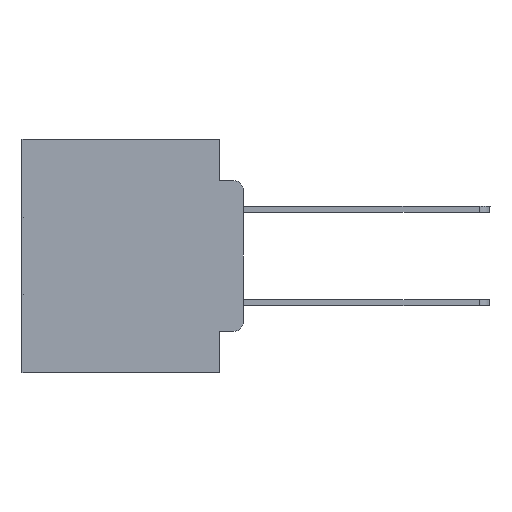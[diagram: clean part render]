
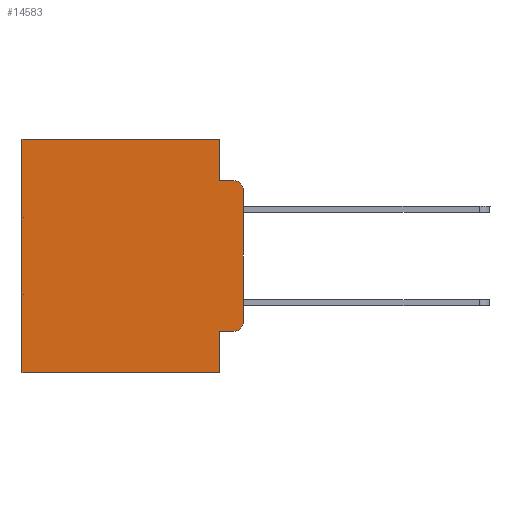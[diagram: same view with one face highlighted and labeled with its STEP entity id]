
A CAD part, left-side view. The second image highlights one B-rep face of the part: STEP entity #14583.
In plain terms, the highlighted planar face has unit normal (-1, 0, 0).
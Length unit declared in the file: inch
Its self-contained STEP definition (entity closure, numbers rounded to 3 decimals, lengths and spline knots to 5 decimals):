
#437 = ORIENTED_EDGE ( 'NONE', *, *, #23579, .T. ) ;
#608 = VECTOR ( 'NONE', #16041, 39.37008 ) ;
#628 = VERTEX_POINT ( 'NONE', #19815 ) ;
#632 = ORIENTED_EDGE ( 'NONE', *, *, #22511, .F. ) ;
#904 = LINE ( 'NONE', #3353, #23796 ) ;
#1685 = ORIENTED_EDGE ( 'NONE', *, *, #5824, .T. ) ;
#2234 = EDGE_CURVE ( 'NONE', #29441, #21208, #904, .T. ) ;
#2269 = ORIENTED_EDGE ( 'NONE', *, *, #23444, .F. ) ;
#2992 = LINE ( 'NONE', #22718, #5276 ) ;
#3216 = VERTEX_POINT ( 'NONE', #29055 ) ;
#3228 = VERTEX_POINT ( 'NONE', #14453 ) ;
#3332 = VERTEX_POINT ( 'NONE', #6909 ) ;
#3353 = CARTESIAN_POINT ( 'NONE',  ( 0.298, 0.051, 0. ) ) ;
#3535 = VECTOR ( 'NONE', #10659, 39.37008 ) ;
#3926 = DIRECTION ( 'NONE',  ( 1., 0., 0. ) ) ;
#4010 = CARTESIAN_POINT ( 'NONE',  ( 0.298, 0., -0.5 ) ) ;
#4019 = CIRCLE ( 'NONE', #18741, 0.02 ) ;
#4032 = CARTESIAN_POINT ( 'NONE',  ( 0.298, 0.02, -0.3915 ) ) ;
#4871 = VERTEX_POINT ( 'NONE', #31496 ) ;
#5253 = EDGE_CURVE ( 'NONE', #29441, #3228, #23105, .T. ) ;
#5276 = VECTOR ( 'NONE', #20769, 39.37008 ) ;
#5824 = EDGE_CURVE ( 'NONE', #3332, #26731, #4019, .T. ) ;
#6003 = DIRECTION ( 'NONE',  ( 0., 0., -1. ) ) ;
#6052 = DIRECTION ( 'NONE',  ( 0., 0., -1. ) ) ;
#6071 = EDGE_CURVE ( 'NONE', #3332, #23024, #2992, .T. ) ;
#6909 = CARTESIAN_POINT ( 'NONE',  ( 0.298, 0., -0.1085 ) ) ;
#7150 = EDGE_CURVE ( 'NONE', #628, #3216, #16087, .T. ) ;
#9857 = CIRCLE ( 'NONE', #19822, 0.02 ) ;
#10036 = ORIENTED_EDGE ( 'NONE', *, *, #7150, .T. ) ;
#10039 = CARTESIAN_POINT ( 'NONE',  ( 0.298, 0.051, -0.5 ) ) ;
#10659 = DIRECTION ( 'NONE',  ( 0., -1., 0. ) ) ;
#11721 = ORIENTED_EDGE ( 'NONE', *, *, #15536, .F. ) ;
#11780 = DIRECTION ( 'NONE',  ( -1., 0., 0. ) ) ;
#12861 = VECTOR ( 'NONE', #19102, 39.37008 ) ;
#13384 = LINE ( 'NONE', #28476, #12861 ) ;
#13494 = VECTOR ( 'NONE', #31547, 39.37008 ) ;
#13768 = DIRECTION ( 'NONE',  ( 0., 0., -1. ) ) ;
#13944 = ORIENTED_EDGE ( 'NONE', *, *, #2234, .F. ) ;
#14076 = VECTOR ( 'NONE', #16365, 39.37008 ) ;
#14153 = EDGE_LOOP ( 'NONE', ( #29452, #1685, #2269, #632, #18569, #10036, #11721, #13944, #29373, #437 ) ) ;
#14453 = CARTESIAN_POINT ( 'NONE',  ( 0.298, 0.02, -0.4115 ) ) ;
#14583 = ADVANCED_FACE ( 'NONE', ( #29064 ), #18916, .F. ) ;
#15536 = EDGE_CURVE ( 'NONE', #21208, #3216, #21444, .T. ) ;
#16041 = DIRECTION ( 'NONE',  ( 0., -1., 0. ) ) ;
#16087 = LINE ( 'NONE', #23145, #21070 ) ;
#16365 = DIRECTION ( 'NONE',  ( 0., 1., 0. ) ) ;
#18569 = ORIENTED_EDGE ( 'NONE', *, *, #20516, .T. ) ;
#18684 = CARTESIAN_POINT ( 'NONE',  ( 0.298, 0.051, -0.0885 ) ) ;
#18741 = AXIS2_PLACEMENT_3D ( 'NONE', #25905, #31010, #6052 ) ;
#18916 = PLANE ( 'NONE',  #28187 ) ;
#19102 = DIRECTION ( 'NONE',  ( 0., 1., 0. ) ) ;
#19372 = CARTESIAN_POINT ( 'NONE',  ( 0.298, 0., -0.3915 ) ) ;
#19815 = CARTESIAN_POINT ( 'NONE',  ( 0.298, 0.473, 0. ) ) ;
#19822 = AXIS2_PLACEMENT_3D ( 'NONE', #4032, #11780, #13768 ) ;
#20516 = EDGE_CURVE ( 'NONE', #4871, #628, #13384, .T. ) ;
#20769 = DIRECTION ( 'NONE',  ( 0., 0., -1. ) ) ;
#21070 = VECTOR ( 'NONE', #21168, 39.37008 ) ;
#21168 = DIRECTION ( 'NONE',  ( 0., 0., -1. ) ) ;
#21208 = VERTEX_POINT ( 'NONE', #10039 ) ;
#21444 = LINE ( 'NONE', #4010, #14076 ) ;
#22511 = EDGE_CURVE ( 'NONE', #4871, #27184, #29567, .T. ) ;
#22718 = CARTESIAN_POINT ( 'NONE',  ( 0.298, 0., 0. ) ) ;
#23024 = VERTEX_POINT ( 'NONE', #19372 ) ;
#23105 = LINE ( 'NONE', #26035, #608 ) ;
#23128 = LINE ( 'NONE', #23279, #3535 ) ;
#23145 = CARTESIAN_POINT ( 'NONE',  ( 0.298, 0.473, 0. ) ) ;
#23279 = CARTESIAN_POINT ( 'NONE',  ( 0.298, 0.051, -0.0885 ) ) ;
#23444 = EDGE_CURVE ( 'NONE', #27184, #26731, #23128, .T. ) ;
#23579 = EDGE_CURVE ( 'NONE', #3228, #23024, #9857, .T. ) ;
#23796 = VECTOR ( 'NONE', #6003, 39.37008 ) ;
#23811 = CARTESIAN_POINT ( 'NONE',  ( 0.298, 0., 0. ) ) ;
#25316 = CARTESIAN_POINT ( 'NONE',  ( 0.298, 0.051, -0.4115 ) ) ;
#25905 = CARTESIAN_POINT ( 'NONE',  ( 0.298, 0.02, -0.1085 ) ) ;
#26035 = CARTESIAN_POINT ( 'NONE',  ( 0.298, 0.051, -0.4115 ) ) ;
#26572 = CARTESIAN_POINT ( 'NONE',  ( 0.298, 0.02, -0.0885 ) ) ;
#26610 = CARTESIAN_POINT ( 'NONE',  ( 0.298, 0.051, 0. ) ) ;
#26731 = VERTEX_POINT ( 'NONE', #26572 ) ;
#27184 = VERTEX_POINT ( 'NONE', #18684 ) ;
#28187 = AXIS2_PLACEMENT_3D ( 'NONE', #23811, #3926, #28912 ) ;
#28476 = CARTESIAN_POINT ( 'NONE',  ( 0.298, 0., 0. ) ) ;
#28912 = DIRECTION ( 'NONE',  ( 0., 0., -1. ) ) ;
#29055 = CARTESIAN_POINT ( 'NONE',  ( 0.298, 0.473, -0.5 ) ) ;
#29064 = FACE_OUTER_BOUND ( 'NONE', #14153, .T. ) ;
#29373 = ORIENTED_EDGE ( 'NONE', *, *, #5253, .T. ) ;
#29441 = VERTEX_POINT ( 'NONE', #25316 ) ;
#29452 = ORIENTED_EDGE ( 'NONE', *, *, #6071, .F. ) ;
#29567 = LINE ( 'NONE', #26610, #13494 ) ;
#31010 = DIRECTION ( 'NONE',  ( -1., 0., 0. ) ) ;
#31496 = CARTESIAN_POINT ( 'NONE',  ( 0.298, 0.051, 0. ) ) ;
#31547 = DIRECTION ( 'NONE',  ( 0., 0., -1. ) ) ;
